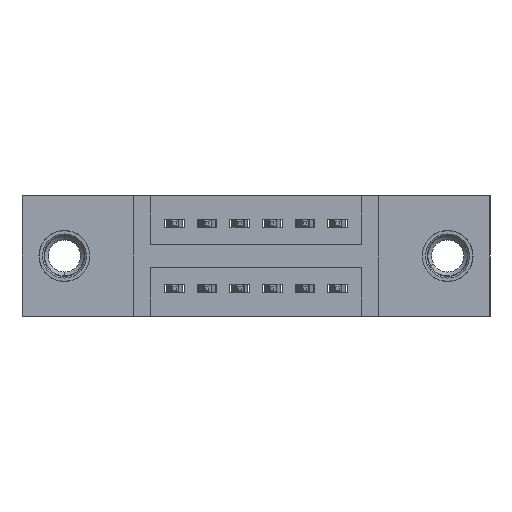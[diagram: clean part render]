
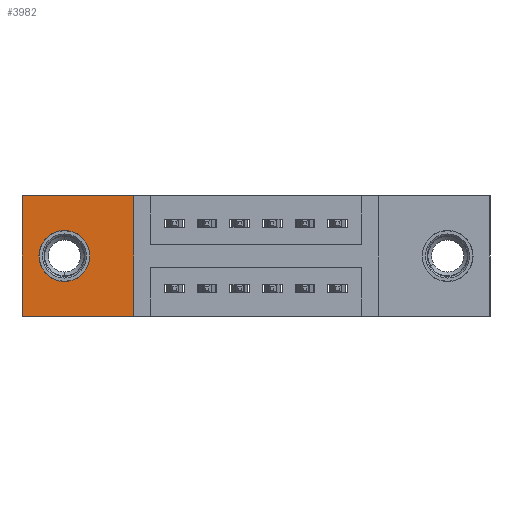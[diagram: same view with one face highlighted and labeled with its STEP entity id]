
A CAD part, front view. The second image highlights one B-rep face of the part: STEP entity #3982.
In plain terms, the highlighted planar face has unit normal (0, -1, 0).
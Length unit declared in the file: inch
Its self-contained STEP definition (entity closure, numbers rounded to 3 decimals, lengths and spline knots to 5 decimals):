
#378 = AXIS2_PLACEMENT_3D ( 'NONE', #1714, #1633, #8468 ) ;
#501 = CARTESIAN_POINT ( 'NONE',  ( 0.13, 0.11, -0.263 ) ) ;
#784 = ORIENTED_EDGE ( 'NONE', *, *, #7714, .F. ) ;
#792 = VERTEX_POINT ( 'NONE', #501 ) ;
#999 = VERTEX_POINT ( 'NONE', #10450 ) ;
#1256 = VECTOR ( 'NONE', #9454, 39.37008 ) ;
#1381 = DIRECTION ( 'NONE',  ( 0., 0., -1. ) ) ;
#1478 = AXIS2_PLACEMENT_3D ( 'NONE', #9152, #4087, #4866 ) ;
#1583 = CARTESIAN_POINT ( 'NONE',  ( 0.3425, 0.11, -0.37 ) ) ;
#1633 = DIRECTION ( 'NONE',  ( 0., -1., 0. ) ) ;
#1714 = CARTESIAN_POINT ( 'NONE',  ( 0., 0.11, -0.37 ) ) ;
#1823 = EDGE_LOOP ( 'NONE', ( #784, #4618 ) ) ;
#2087 = DIRECTION ( 'NONE',  ( 0., 0., -1. ) ) ;
#2120 = CIRCLE ( 'NONE', #9692, 0.078 ) ;
#2175 = CARTESIAN_POINT ( 'NONE',  ( 0., 0.11, 0. ) ) ;
#2764 = DIRECTION ( 'NONE',  ( 0., 0., 1. ) ) ;
#2891 = CARTESIAN_POINT ( 'NONE',  ( 0., 0.11, -0.37 ) ) ;
#2968 = FACE_BOUND ( 'NONE', #1823, .T. ) ;
#3344 = EDGE_CURVE ( 'NONE', #6075, #4097, #10389, .T. ) ;
#3392 = EDGE_LOOP ( 'NONE', ( #4900, #8880, #8911, #6606 ) ) ;
#3899 = VERTEX_POINT ( 'NONE', #4880 ) ;
#3982 = ADVANCED_FACE ( 'NONE', ( #2968, #4556 ), #10891, .T. ) ;
#4087 = DIRECTION ( 'NONE',  ( 0., -1., 0. ) ) ;
#4097 = VERTEX_POINT ( 'NONE', #2891 ) ;
#4412 = CARTESIAN_POINT ( 'NONE',  ( 0.3425, 0.11, 0. ) ) ;
#4556 = FACE_OUTER_BOUND ( 'NONE', #3392, .T. ) ;
#4566 = LINE ( 'NONE', #4412, #10771 ) ;
#4618 = ORIENTED_EDGE ( 'NONE', *, *, #5706, .F. ) ;
#4789 = CIRCLE ( 'NONE', #1478, 0.078 ) ;
#4810 = CARTESIAN_POINT ( 'NONE',  ( 0., 0.11, 0. ) ) ;
#4866 = DIRECTION ( 'NONE',  ( 0., 0., -1. ) ) ;
#4880 = CARTESIAN_POINT ( 'NONE',  ( 0.13, 0.11, -0.107 ) ) ;
#4890 = EDGE_CURVE ( 'NONE', #4097, #5213, #6674, .T. ) ;
#4900 = ORIENTED_EDGE ( 'NONE', *, *, #3344, .T. ) ;
#5213 = VERTEX_POINT ( 'NONE', #1583 ) ;
#5706 = EDGE_CURVE ( 'NONE', #792, #3899, #4789, .T. ) ;
#6075 = VERTEX_POINT ( 'NONE', #9328 ) ;
#6606 = ORIENTED_EDGE ( 'NONE', *, *, #7305, .T. ) ;
#6674 = LINE ( 'NONE', #10274, #1256 ) ;
#7157 = DIRECTION ( 'NONE',  ( -1., 0., 0. ) ) ;
#7305 = EDGE_CURVE ( 'NONE', #999, #6075, #10840, .T. ) ;
#7684 = VECTOR ( 'NONE', #7157, 39.37008 ) ;
#7714 = EDGE_CURVE ( 'NONE', #3899, #792, #2120, .T. ) ;
#8468 = DIRECTION ( 'NONE',  ( 0., 0., -1. ) ) ;
#8792 = DIRECTION ( 'NONE',  ( 0., -1., 0. ) ) ;
#8880 = ORIENTED_EDGE ( 'NONE', *, *, #4890, .T. ) ;
#8911 = ORIENTED_EDGE ( 'NONE', *, *, #10337, .T. ) ;
#9152 = CARTESIAN_POINT ( 'NONE',  ( 0.13, 0.11, -0.185 ) ) ;
#9328 = CARTESIAN_POINT ( 'NONE',  ( 0., 0.11, 0. ) ) ;
#9454 = DIRECTION ( 'NONE',  ( 1., 0., 0. ) ) ;
#9565 = CARTESIAN_POINT ( 'NONE',  ( 0.13, 0.11, -0.185 ) ) ;
#9692 = AXIS2_PLACEMENT_3D ( 'NONE', #9565, #8792, #2087 ) ;
#10274 = CARTESIAN_POINT ( 'NONE',  ( 0., 0.11, -0.37 ) ) ;
#10337 = EDGE_CURVE ( 'NONE', #5213, #999, #4566, .T. ) ;
#10389 = LINE ( 'NONE', #4810, #10647 ) ;
#10450 = CARTESIAN_POINT ( 'NONE',  ( 0.3425, 0.11, 0. ) ) ;
#10647 = VECTOR ( 'NONE', #1381, 39.37008 ) ;
#10771 = VECTOR ( 'NONE', #2764, 39.37008 ) ;
#10840 = LINE ( 'NONE', #2175, #7684 ) ;
#10891 = PLANE ( 'NONE',  #378 ) ;
